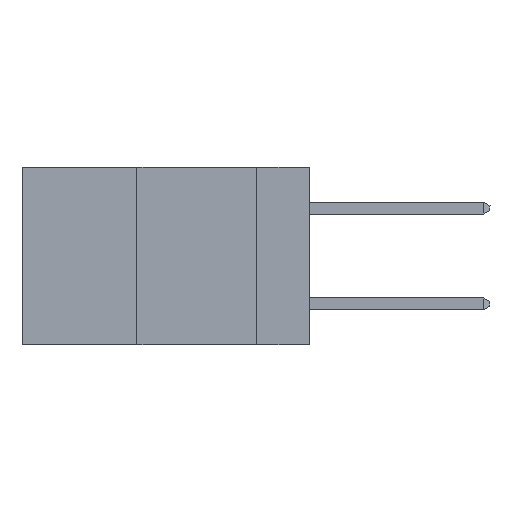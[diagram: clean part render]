
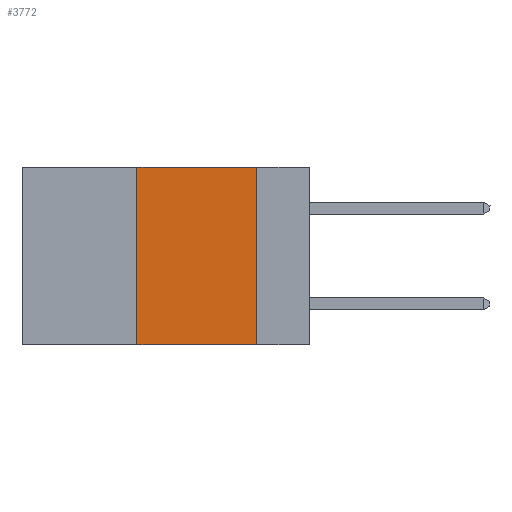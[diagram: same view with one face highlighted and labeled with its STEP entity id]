
A CAD part, left-side view. The second image highlights one B-rep face of the part: STEP entity #3772.
In plain terms, the highlighted planar face has unit normal (-1, 0, 0).
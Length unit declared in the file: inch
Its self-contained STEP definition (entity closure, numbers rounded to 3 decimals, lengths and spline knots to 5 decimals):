
#1389 = VECTOR ( 'NONE', #5474, 39.37008 ) ;
#1732 = EDGE_CURVE ( 'NONE', #8879, #4830, #9110, .T. ) ;
#2575 = AXIS2_PLACEMENT_3D ( 'NONE', #4732, #5215, #7270 ) ;
#2679 = DIRECTION ( 'NONE',  ( 0., -1., 0. ) ) ;
#2781 = DIRECTION ( 'NONE',  ( 0., 0., -1. ) ) ;
#2828 = ORIENTED_EDGE ( 'NONE', *, *, #8719, .F. ) ;
#2849 = VERTEX_POINT ( 'NONE', #4878 ) ;
#3667 = ORIENTED_EDGE ( 'NONE', *, *, #1732, .F. ) ;
#3772 = ADVANCED_FACE ( 'NONE', ( #9562 ), #4705, .F. ) ;
#3803 = ORIENTED_EDGE ( 'NONE', *, *, #7646, .F. ) ;
#4037 = ORIENTED_EDGE ( 'NONE', *, *, #6476, .T. ) ;
#4198 = CARTESIAN_POINT ( 'NONE',  ( 0., 0.6, 0. ) ) ;
#4705 = PLANE ( 'NONE',  #2575 ) ;
#4732 = CARTESIAN_POINT ( 'NONE',  ( 0., 0.6, 0. ) ) ;
#4748 = CARTESIAN_POINT ( 'NONE',  ( 0., 0.36, 0. ) ) ;
#4812 = LINE ( 'NONE', #6731, #9509 ) ;
#4830 = VERTEX_POINT ( 'NONE', #8110 ) ;
#4878 = CARTESIAN_POINT ( 'NONE',  ( 0., 0.11, -0.37 ) ) ;
#5215 = DIRECTION ( 'NONE',  ( 1., 0., 0. ) ) ;
#5412 = VECTOR ( 'NONE', #2679, 39.37008 ) ;
#5474 = DIRECTION ( 'NONE',  ( 0., 0., 1. ) ) ;
#5577 = VECTOR ( 'NONE', #7626, 39.37008 ) ;
#6476 = EDGE_CURVE ( 'NONE', #9324, #2849, #7421, .T. ) ;
#6616 = CARTESIAN_POINT ( 'NONE',  ( 0., 0.6, -0.37 ) ) ;
#6731 = CARTESIAN_POINT ( 'NONE',  ( 0., 0.11, 0. ) ) ;
#7270 = DIRECTION ( 'NONE',  ( 0., 0., -1. ) ) ;
#7421 = LINE ( 'NONE', #6616, #5412 ) ;
#7626 = DIRECTION ( 'NONE',  ( 0., -1., 0. ) ) ;
#7628 = CARTESIAN_POINT ( 'NONE',  ( 0., 0.36, -0.37 ) ) ;
#7646 = EDGE_CURVE ( 'NONE', #4830, #2849, #4812, .T. ) ;
#7998 = LINE ( 'NONE', #4748, #1389 ) ;
#8110 = CARTESIAN_POINT ( 'NONE',  ( 0., 0.11, 0. ) ) ;
#8461 = CARTESIAN_POINT ( 'NONE',  ( 0., 0.36, 0. ) ) ;
#8719 = EDGE_CURVE ( 'NONE', #9324, #8879, #7998, .T. ) ;
#8879 = VERTEX_POINT ( 'NONE', #8461 ) ;
#9110 = LINE ( 'NONE', #4198, #5577 ) ;
#9324 = VERTEX_POINT ( 'NONE', #7628 ) ;
#9508 = EDGE_LOOP ( 'NONE', ( #3803, #3667, #2828, #4037 ) ) ;
#9509 = VECTOR ( 'NONE', #2781, 39.37008 ) ;
#9562 = FACE_OUTER_BOUND ( 'NONE', #9508, .T. ) ;
